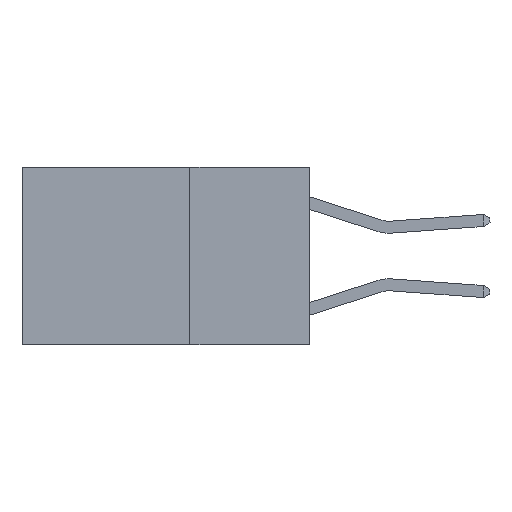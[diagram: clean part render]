
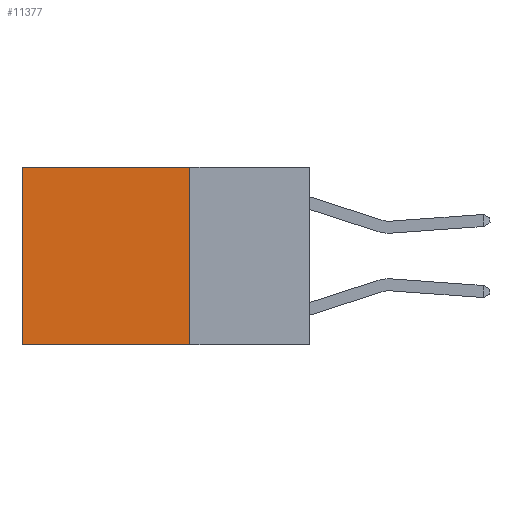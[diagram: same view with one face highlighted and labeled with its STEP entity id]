
A CAD part, left-side view. The second image highlights one B-rep face of the part: STEP entity #11377.
In plain terms, the highlighted planar face has unit normal (-1, 0, 0).
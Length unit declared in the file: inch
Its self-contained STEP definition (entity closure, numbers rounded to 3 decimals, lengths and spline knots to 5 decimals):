
#51 = EDGE_CURVE ( 'NONE', #9231, #2594, #17901, .T. ) ;
#2247 = EDGE_CURVE ( 'NONE', #18309, #2594, #7203, .T. ) ;
#2594 = VERTEX_POINT ( 'NONE', #19093 ) ;
#2708 = VECTOR ( 'NONE', #7055, 39.37008 ) ;
#2870 = DIRECTION ( 'NONE',  ( 0., 1., 0. ) ) ;
#2875 = CARTESIAN_POINT ( 'NONE',  ( 0.2625, 0.25, 0. ) ) ;
#3432 = LINE ( 'NONE', #15510, #17755 ) ;
#3810 = LINE ( 'NONE', #17223, #2708 ) ;
#3854 = ORIENTED_EDGE ( 'NONE', *, *, #51, .T. ) ;
#4231 = CARTESIAN_POINT ( 'NONE',  ( 0.2625, 0.25, 0. ) ) ;
#4728 = AXIS2_PLACEMENT_3D ( 'NONE', #4231, #16310, #14318 ) ;
#6669 = VECTOR ( 'NONE', #2870, 39.37008 ) ;
#7055 = DIRECTION ( 'NONE',  ( 0., 1., 0. ) ) ;
#7203 = LINE ( 'NONE', #17857, #6669 ) ;
#8054 = EDGE_LOOP ( 'NONE', ( #3854, #16437, #20134, #11437 ) ) ;
#8278 = CARTESIAN_POINT ( 'NONE',  ( 0.2625, 0.6, 0. ) ) ;
#8719 = CARTESIAN_POINT ( 'NONE',  ( 0.2625, 0.6, 0. ) ) ;
#9231 = VERTEX_POINT ( 'NONE', #8278 ) ;
#10762 = VECTOR ( 'NONE', #20527, 39.37008 ) ;
#11377 = ADVANCED_FACE ( 'NONE', ( #21096 ), #14396, .F. ) ;
#11437 = ORIENTED_EDGE ( 'NONE', *, *, #12400, .T. ) ;
#12400 = EDGE_CURVE ( 'NONE', #21150, #9231, #3810, .T. ) ;
#14318 = DIRECTION ( 'NONE',  ( 0., 0., -1. ) ) ;
#14396 = PLANE ( 'NONE',  #4728 ) ;
#15510 = CARTESIAN_POINT ( 'NONE',  ( 0.2625, 0.25, 0. ) ) ;
#16310 = DIRECTION ( 'NONE',  ( 1., 0., 0. ) ) ;
#16437 = ORIENTED_EDGE ( 'NONE', *, *, #2247, .F. ) ;
#17223 = CARTESIAN_POINT ( 'NONE',  ( 0.2625, 0.25, 0. ) ) ;
#17755 = VECTOR ( 'NONE', #20635, 39.37008 ) ;
#17857 = CARTESIAN_POINT ( 'NONE',  ( 0.2625, 0.25, -0.37 ) ) ;
#17901 = LINE ( 'NONE', #8719, #10762 ) ;
#18309 = VERTEX_POINT ( 'NONE', #20614 ) ;
#19093 = CARTESIAN_POINT ( 'NONE',  ( 0.2625, 0.6, -0.37 ) ) ;
#20134 = ORIENTED_EDGE ( 'NONE', *, *, #20775, .F. ) ;
#20527 = DIRECTION ( 'NONE',  ( 0., 0., -1. ) ) ;
#20614 = CARTESIAN_POINT ( 'NONE',  ( 0.2625, 0.25, -0.37 ) ) ;
#20635 = DIRECTION ( 'NONE',  ( 0., 0., -1. ) ) ;
#20775 = EDGE_CURVE ( 'NONE', #21150, #18309, #3432, .T. ) ;
#21096 = FACE_OUTER_BOUND ( 'NONE', #8054, .T. ) ;
#21150 = VERTEX_POINT ( 'NONE', #2875 ) ;
